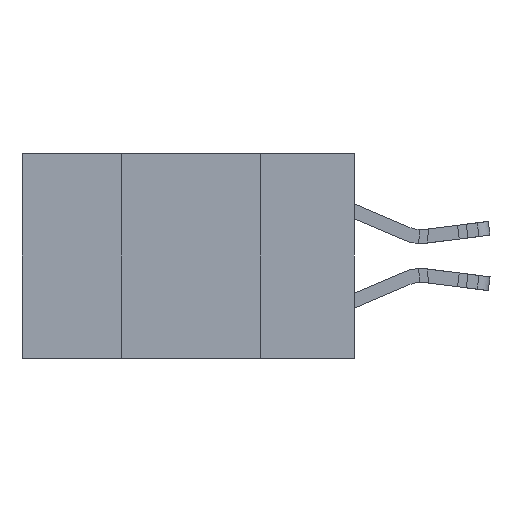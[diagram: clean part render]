
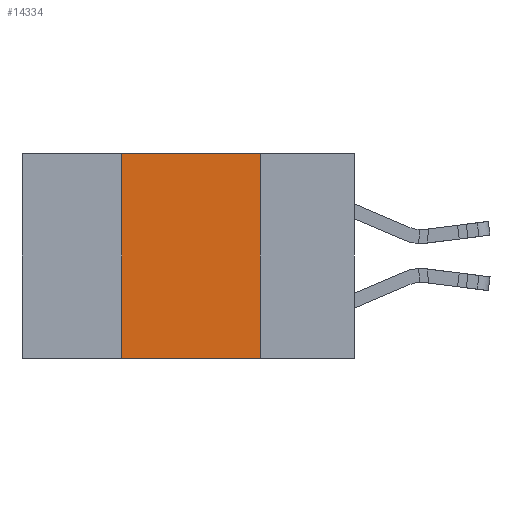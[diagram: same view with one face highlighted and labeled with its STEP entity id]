
A CAD part, left-side view. The second image highlights one B-rep face of the part: STEP entity #14334.
In plain terms, the highlighted planar face has unit normal (-1, 0, 0).
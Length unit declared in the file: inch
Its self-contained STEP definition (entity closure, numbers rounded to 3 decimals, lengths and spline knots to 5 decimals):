
#874 = DIRECTION ( 'NONE',  ( 1., 0., 0. ) ) ;
#1350 = LINE ( 'NONE', #1868, #22138 ) ;
#1868 = CARTESIAN_POINT ( 'NONE',  ( 0., 0.6, 0. ) ) ;
#2091 = DIRECTION ( 'NONE',  ( 0., -1., 0. ) ) ;
#2381 = VERTEX_POINT ( 'NONE', #3704 ) ;
#2490 = LINE ( 'NONE', #5355, #32640 ) ;
#3038 = CARTESIAN_POINT ( 'NONE',  ( 0., 0.42, 0. ) ) ;
#3704 = CARTESIAN_POINT ( 'NONE',  ( 0., 0.42, -0.37 ) ) ;
#4814 = EDGE_CURVE ( 'NONE', #16980, #19266, #1350, .T. ) ;
#5273 = LINE ( 'NONE', #16993, #18372 ) ;
#5355 = CARTESIAN_POINT ( 'NONE',  ( 0., 0.42, 0. ) ) ;
#5560 = EDGE_CURVE ( 'NONE', #19266, #23345, #18035, .T. ) ;
#5960 = DIRECTION ( 'NONE',  ( 0., 0., -1. ) ) ;
#6184 = CARTESIAN_POINT ( 'NONE',  ( 0., 0.6, 0. ) ) ;
#7978 = AXIS2_PLACEMENT_3D ( 'NONE', #6184, #874, #16621 ) ;
#8209 = VECTOR ( 'NONE', #5960, 39.37008 ) ;
#13686 = CARTESIAN_POINT ( 'NONE',  ( 0., 0.17, 0. ) ) ;
#14334 = ADVANCED_FACE ( 'NONE', ( #15972 ), #32505, .F. ) ;
#14865 = ORIENTED_EDGE ( 'NONE', *, *, #4814, .F. ) ;
#15972 = FACE_OUTER_BOUND ( 'NONE', #33523, .T. ) ;
#16621 = DIRECTION ( 'NONE',  ( 0., 0., -1. ) ) ;
#16980 = VERTEX_POINT ( 'NONE', #3038 ) ;
#16993 = CARTESIAN_POINT ( 'NONE',  ( 0., 0.6, -0.37 ) ) ;
#18035 = LINE ( 'NONE', #13686, #8209 ) ;
#18372 = VECTOR ( 'NONE', #27190, 39.37008 ) ;
#18694 = ORIENTED_EDGE ( 'NONE', *, *, #5560, .F. ) ;
#19119 = CARTESIAN_POINT ( 'NONE',  ( 0., 0.17, -0.37 ) ) ;
#19266 = VERTEX_POINT ( 'NONE', #22053 ) ;
#19968 = ORIENTED_EDGE ( 'NONE', *, *, #33129, .T. ) ;
#22053 = CARTESIAN_POINT ( 'NONE',  ( 0., 0.17, 0. ) ) ;
#22138 = VECTOR ( 'NONE', #2091, 39.37008 ) ;
#23345 = VERTEX_POINT ( 'NONE', #19119 ) ;
#23601 = DIRECTION ( 'NONE',  ( 0., 0., 1. ) ) ;
#27190 = DIRECTION ( 'NONE',  ( 0., -1., 0. ) ) ;
#27722 = ORIENTED_EDGE ( 'NONE', *, *, #29300, .F. ) ;
#29300 = EDGE_CURVE ( 'NONE', #2381, #16980, #2490, .T. ) ;
#32505 = PLANE ( 'NONE',  #7978 ) ;
#32640 = VECTOR ( 'NONE', #23601, 39.37008 ) ;
#33129 = EDGE_CURVE ( 'NONE', #2381, #23345, #5273, .T. ) ;
#33523 = EDGE_LOOP ( 'NONE', ( #18694, #14865, #27722, #19968 ) ) ;
